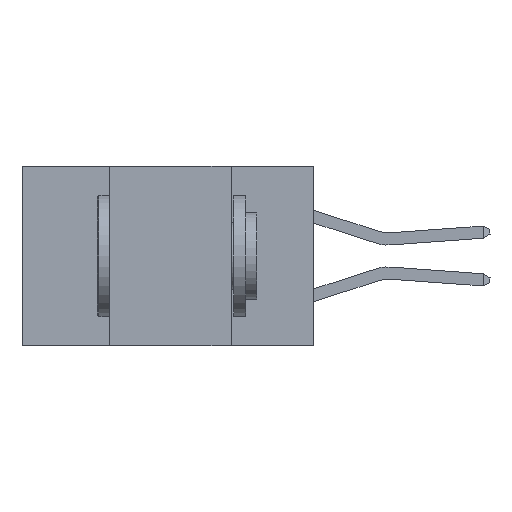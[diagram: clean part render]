
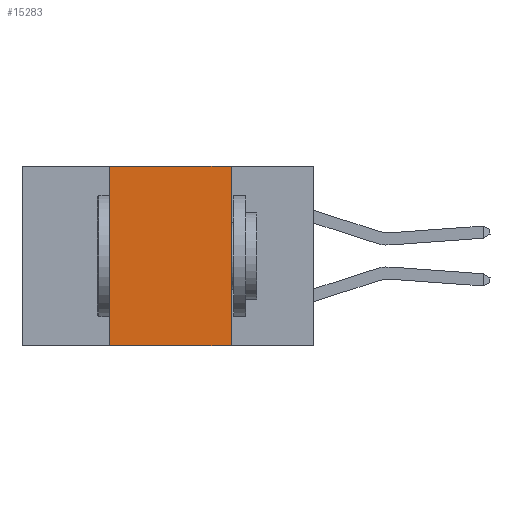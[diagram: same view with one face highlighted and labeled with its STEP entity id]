
A CAD part, left-side view. The second image highlights one B-rep face of the part: STEP entity #15283.
In plain terms, the highlighted planar face has unit normal (-1, 0, 0).
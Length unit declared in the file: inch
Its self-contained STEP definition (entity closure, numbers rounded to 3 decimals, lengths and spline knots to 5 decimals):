
#32 = LINE ( 'NONE', #9830, #28278 ) ;
#3286 = DIRECTION ( 'NONE',  ( 0., -1., 0. ) ) ;
#4436 = DIRECTION ( 'NONE',  ( 0., 0., -1. ) ) ;
#5409 = DIRECTION ( 'NONE',  ( 1., 0., 0. ) ) ;
#7501 = ORIENTED_EDGE ( 'NONE', *, *, #25185, .F. ) ;
#7543 = FACE_OUTER_BOUND ( 'NONE', #17817, .T. ) ;
#8072 = AXIS2_PLACEMENT_3D ( 'NONE', #10824, #5409, #24479 ) ;
#9830 = CARTESIAN_POINT ( 'NONE',  ( 0., 0.6, 0. ) ) ;
#10007 = VECTOR ( 'NONE', #3286, 39.37008 ) ;
#10824 = CARTESIAN_POINT ( 'NONE',  ( 0., 0.6, 0. ) ) ;
#10873 = LINE ( 'NONE', #11487, #10007 ) ;
#11380 = VERTEX_POINT ( 'NONE', #13457 ) ;
#11487 = CARTESIAN_POINT ( 'NONE',  ( 0., 0.6, -0.37 ) ) ;
#12073 = CARTESIAN_POINT ( 'NONE',  ( 0., 0.42, 0. ) ) ;
#12564 = CARTESIAN_POINT ( 'NONE',  ( 0., 0.17, 0. ) ) ;
#13331 = VERTEX_POINT ( 'NONE', #16173 ) ;
#13457 = CARTESIAN_POINT ( 'NONE',  ( 0., 0.17, 0. ) ) ;
#14782 = DIRECTION ( 'NONE',  ( 0., 0., 1. ) ) ;
#14898 = CARTESIAN_POINT ( 'NONE',  ( 0., 0.42, -0.37 ) ) ;
#15283 = ADVANCED_FACE ( 'NONE', ( #7543 ), #21747, .F. ) ;
#15720 = EDGE_CURVE ( 'NONE', #16762, #11380, #32, .T. ) ;
#16173 = CARTESIAN_POINT ( 'NONE',  ( 0., 0.17, -0.37 ) ) ;
#16762 = VERTEX_POINT ( 'NONE', #17861 ) ;
#17817 = EDGE_LOOP ( 'NONE', ( #7501, #29457, #23668, #20247 ) ) ;
#17861 = CARTESIAN_POINT ( 'NONE',  ( 0., 0.42, 0. ) ) ;
#19434 = VECTOR ( 'NONE', #14782, 39.37008 ) ;
#20247 = ORIENTED_EDGE ( 'NONE', *, *, #20385, .T. ) ;
#20385 = EDGE_CURVE ( 'NONE', #20586, #13331, #10873, .T. ) ;
#20586 = VERTEX_POINT ( 'NONE', #14898 ) ;
#21747 = PLANE ( 'NONE',  #8072 ) ;
#23122 = VECTOR ( 'NONE', #4436, 39.37008 ) ;
#23668 = ORIENTED_EDGE ( 'NONE', *, *, #31138, .F. ) ;
#24479 = DIRECTION ( 'NONE',  ( 0., 0., -1. ) ) ;
#25185 = EDGE_CURVE ( 'NONE', #11380, #13331, #31033, .T. ) ;
#28278 = VECTOR ( 'NONE', #34027, 39.37008 ) ;
#29457 = ORIENTED_EDGE ( 'NONE', *, *, #15720, .F. ) ;
#31033 = LINE ( 'NONE', #12564, #23122 ) ;
#31138 = EDGE_CURVE ( 'NONE', #20586, #16762, #33611, .T. ) ;
#33611 = LINE ( 'NONE', #12073, #19434 ) ;
#34027 = DIRECTION ( 'NONE',  ( 0., -1., 0. ) ) ;
